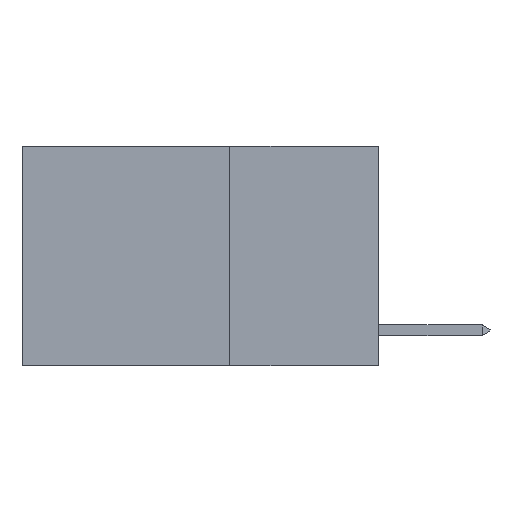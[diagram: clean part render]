
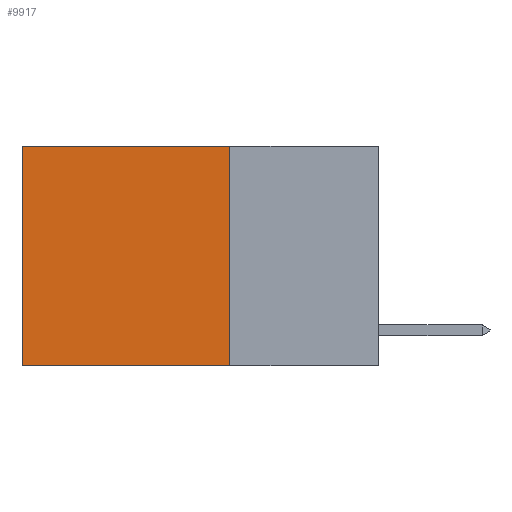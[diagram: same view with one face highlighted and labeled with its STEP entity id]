
A CAD part, left-side view. The second image highlights one B-rep face of the part: STEP entity #9917.
In plain terms, the highlighted planar face has unit normal (-1, 0, 0).
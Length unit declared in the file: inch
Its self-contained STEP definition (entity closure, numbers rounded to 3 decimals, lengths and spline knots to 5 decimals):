
#397 = DIRECTION ( 'NONE',  ( 0., 0., -1. ) ) ;
#507 = DIRECTION ( 'NONE',  ( 0., 0., -1. ) ) ;
#708 = CARTESIAN_POINT ( 'NONE',  ( 0.2625, 0.25, 0. ) ) ;
#1461 = LINE ( 'NONE', #4122, #14639 ) ;
#2181 = CARTESIAN_POINT ( 'NONE',  ( 0.2625, 0.25, -0.37 ) ) ;
#2287 = EDGE_CURVE ( 'NONE', #3437, #15732, #4902, .T. ) ;
#3146 = PLANE ( 'NONE',  #14236 ) ;
#3437 = VERTEX_POINT ( 'NONE', #6193 ) ;
#3579 = EDGE_CURVE ( 'NONE', #13347, #4944, #5593, .T. ) ;
#4094 = EDGE_CURVE ( 'NONE', #13347, #3437, #1461, .T. ) ;
#4122 = CARTESIAN_POINT ( 'NONE',  ( 0.2625, 0.25, 0. ) ) ;
#4429 = CARTESIAN_POINT ( 'NONE',  ( 0.2625, 0.25, -0.37 ) ) ;
#4902 = LINE ( 'NONE', #10139, #10333 ) ;
#4944 = VERTEX_POINT ( 'NONE', #2181 ) ;
#5593 = LINE ( 'NONE', #14412, #9472 ) ;
#6103 = DIRECTION ( 'NONE',  ( 0., 0., -1. ) ) ;
#6193 = CARTESIAN_POINT ( 'NONE',  ( 0.2625, 0.6, 0. ) ) ;
#7675 = ORIENTED_EDGE ( 'NONE', *, *, #16801, .F. ) ;
#8196 = DIRECTION ( 'NONE',  ( 0., 1., 0. ) ) ;
#8909 = VECTOR ( 'NONE', #8196, 39.37008 ) ;
#9201 = ORIENTED_EDGE ( 'NONE', *, *, #2287, .T. ) ;
#9472 = VECTOR ( 'NONE', #397, 39.37008 ) ;
#9560 = FACE_OUTER_BOUND ( 'NONE', #11025, .T. ) ;
#9903 = ORIENTED_EDGE ( 'NONE', *, *, #4094, .T. ) ;
#9917 = ADVANCED_FACE ( 'NONE', ( #9560 ), #3146, .F. ) ;
#10139 = CARTESIAN_POINT ( 'NONE',  ( 0.2625, 0.6, 0. ) ) ;
#10333 = VECTOR ( 'NONE', #6103, 39.37008 ) ;
#11025 = EDGE_LOOP ( 'NONE', ( #9201, #7675, #11130, #9903 ) ) ;
#11130 = ORIENTED_EDGE ( 'NONE', *, *, #3579, .F. ) ;
#11205 = DIRECTION ( 'NONE',  ( 1., 0., 0. ) ) ;
#12519 = DIRECTION ( 'NONE',  ( 0., 1., 0. ) ) ;
#13347 = VERTEX_POINT ( 'NONE', #708 ) ;
#14236 = AXIS2_PLACEMENT_3D ( 'NONE', #14964, #11205, #507 ) ;
#14412 = CARTESIAN_POINT ( 'NONE',  ( 0.2625, 0.25, 0. ) ) ;
#14639 = VECTOR ( 'NONE', #12519, 39.37008 ) ;
#14742 = CARTESIAN_POINT ( 'NONE',  ( 0.2625, 0.6, -0.37 ) ) ;
#14964 = CARTESIAN_POINT ( 'NONE',  ( 0.2625, 0.25, 0. ) ) ;
#15049 = LINE ( 'NONE', #4429, #8909 ) ;
#15732 = VERTEX_POINT ( 'NONE', #14742 ) ;
#16801 = EDGE_CURVE ( 'NONE', #4944, #15732, #15049, .T. ) ;
